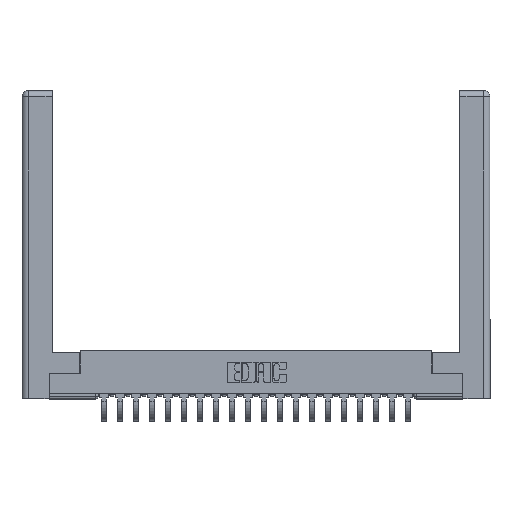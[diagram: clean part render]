
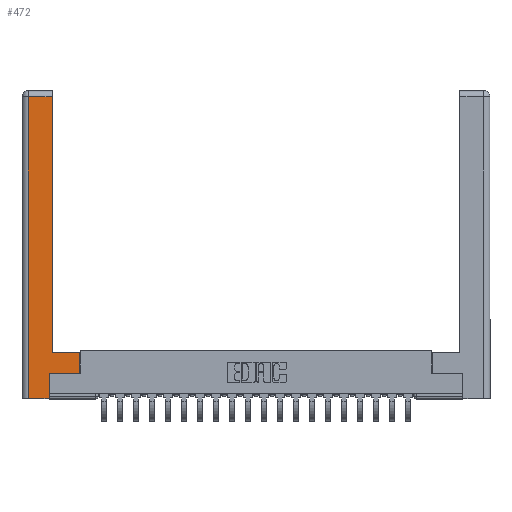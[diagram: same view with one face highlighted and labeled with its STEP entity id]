
A CAD part, top view. The second image highlights one B-rep face of the part: STEP entity #472.
In plain terms, the highlighted planar face has unit normal (0, 0, 1).
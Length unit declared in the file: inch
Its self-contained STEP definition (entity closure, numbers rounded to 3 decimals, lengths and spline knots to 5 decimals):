
#187 = CARTESIAN_POINT ( 'NONE',  ( 0.265, 0.245, 0. ) ) ;
#472 = ADVANCED_FACE ( 'NONE', ( #3851 ), #8752, .F. ) ;
#750 = CARTESIAN_POINT ( 'NONE',  ( 0.295, 0.45, 0. ) ) ;
#1135 = DIRECTION ( 'NONE',  ( 0., -1., 0. ) ) ;
#2052 = CARTESIAN_POINT ( 'NONE',  ( 0.565, 0.45, 0. ) ) ;
#2183 = LINE ( 'NONE', #187, #10920 ) ;
#2448 = ORIENTED_EDGE ( 'NONE', *, *, #23959, .T. ) ;
#2624 = VERTEX_POINT ( 'NONE', #21169 ) ;
#2901 = DIRECTION ( 'NONE',  ( 0., 1., 0. ) ) ;
#3128 = LINE ( 'NONE', #18568, #22253 ) ;
#3155 = EDGE_CURVE ( 'NONE', #6055, #11243, #2183, .T. ) ;
#3174 = VERTEX_POINT ( 'NONE', #2052 ) ;
#3216 = VERTEX_POINT ( 'NONE', #20635 ) ;
#3851 = FACE_OUTER_BOUND ( 'NONE', #22359, .T. ) ;
#3997 = DIRECTION ( 'NONE',  ( 1., 0., 0. ) ) ;
#4145 = LINE ( 'NONE', #13250, #11131 ) ;
#4746 = CARTESIAN_POINT ( 'NONE',  ( 0.265, 0., 0. ) ) ;
#5185 = EDGE_CURVE ( 'NONE', #3216, #6055, #22564, .T. ) ;
#5378 = CARTESIAN_POINT ( 'NONE',  ( 0.0615, 2.94, 0. ) ) ;
#6015 = DIRECTION ( 'NONE',  ( 0., 1., 0. ) ) ;
#6055 = VERTEX_POINT ( 'NONE', #4746 ) ;
#6463 = CARTESIAN_POINT ( 'NONE',  ( 0.295, 0.45, 0. ) ) ;
#7037 = VERTEX_POINT ( 'NONE', #5378 ) ;
#7240 = EDGE_CURVE ( 'NONE', #2624, #7037, #15851, .T. ) ;
#7978 = CARTESIAN_POINT ( 'NONE',  ( 0.565, 0.245, 0. ) ) ;
#8579 = DIRECTION ( 'NONE',  ( -1., 0., 0. ) ) ;
#8752 = PLANE ( 'NONE',  #8861 ) ;
#8769 = ORIENTED_EDGE ( 'NONE', *, *, #16423, .T. ) ;
#8861 = AXIS2_PLACEMENT_3D ( 'NONE', #13211, #13336, #16368 ) ;
#9032 = VERTEX_POINT ( 'NONE', #750 ) ;
#9096 = ORIENTED_EDGE ( 'NONE', *, *, #10620, .T. ) ;
#9482 = VECTOR ( 'NONE', #3997, 39.37008 ) ;
#9861 = DIRECTION ( 'NONE',  ( -1., 0., 0. ) ) ;
#10332 = LINE ( 'NONE', #6463, #16298 ) ;
#10620 = EDGE_CURVE ( 'NONE', #11243, #18313, #19334, .T. ) ;
#10920 = VECTOR ( 'NONE', #15384, 39.37008 ) ;
#11131 = VECTOR ( 'NONE', #6015, 39.37008 ) ;
#11243 = VERTEX_POINT ( 'NONE', #12172 ) ;
#11342 = CARTESIAN_POINT ( 'NONE',  ( 0.265, 0., 0. ) ) ;
#12172 = CARTESIAN_POINT ( 'NONE',  ( 0.265, 0.245, 0. ) ) ;
#13192 = VECTOR ( 'NONE', #2901, 39.37008 ) ;
#13211 = CARTESIAN_POINT ( 'NONE',  ( 0., 0., 0. ) ) ;
#13250 = CARTESIAN_POINT ( 'NONE',  ( 0.565, 0.45, 0. ) ) ;
#13336 = DIRECTION ( 'NONE',  ( 0., 0., -1. ) ) ;
#13463 = ORIENTED_EDGE ( 'NONE', *, *, #22602, .T. ) ;
#14272 = ORIENTED_EDGE ( 'NONE', *, *, #16146, .T. ) ;
#14895 = ORIENTED_EDGE ( 'NONE', *, *, #5185, .T. ) ;
#15384 = DIRECTION ( 'NONE',  ( 0., 1., 0. ) ) ;
#15851 = LINE ( 'NONE', #17728, #18065 ) ;
#16146 = EDGE_CURVE ( 'NONE', #7037, #3216, #3128, .T. ) ;
#16298 = VECTOR ( 'NONE', #8579, 39.37008 ) ;
#16368 = DIRECTION ( 'NONE',  ( -1., 0., 0. ) ) ;
#16423 = EDGE_CURVE ( 'NONE', #3174, #9032, #10332, .T. ) ;
#16827 = DIRECTION ( 'NONE',  ( 1., 0., 0. ) ) ;
#17026 = VECTOR ( 'NONE', #16827, 39.37008 ) ;
#17728 = CARTESIAN_POINT ( 'NONE',  ( 0.0615, 2.94, 0. ) ) ;
#17863 = CARTESIAN_POINT ( 'NONE',  ( 0.295, 3., 0. ) ) ;
#18065 = VECTOR ( 'NONE', #9861, 39.37008 ) ;
#18313 = VERTEX_POINT ( 'NONE', #20033 ) ;
#18568 = CARTESIAN_POINT ( 'NONE',  ( 0.0615, 0., 0. ) ) ;
#19334 = LINE ( 'NONE', #7978, #9482 ) ;
#19464 = ORIENTED_EDGE ( 'NONE', *, *, #3155, .T. ) ;
#20033 = CARTESIAN_POINT ( 'NONE',  ( 0.565, 0.245, 0. ) ) ;
#20635 = CARTESIAN_POINT ( 'NONE',  ( 0.0615, 0., 0. ) ) ;
#21169 = CARTESIAN_POINT ( 'NONE',  ( 0.295, 2.94, 0. ) ) ;
#21737 = LINE ( 'NONE', #17863, #13192 ) ;
#22253 = VECTOR ( 'NONE', #1135, 39.37008 ) ;
#22359 = EDGE_LOOP ( 'NONE', ( #2448, #22788, #14272, #14895, #19464, #9096, #13463, #8769 ) ) ;
#22564 = LINE ( 'NONE', #11342, #17026 ) ;
#22602 = EDGE_CURVE ( 'NONE', #18313, #3174, #4145, .T. ) ;
#22788 = ORIENTED_EDGE ( 'NONE', *, *, #7240, .T. ) ;
#23959 = EDGE_CURVE ( 'NONE', #9032, #2624, #21737, .T. ) ;
